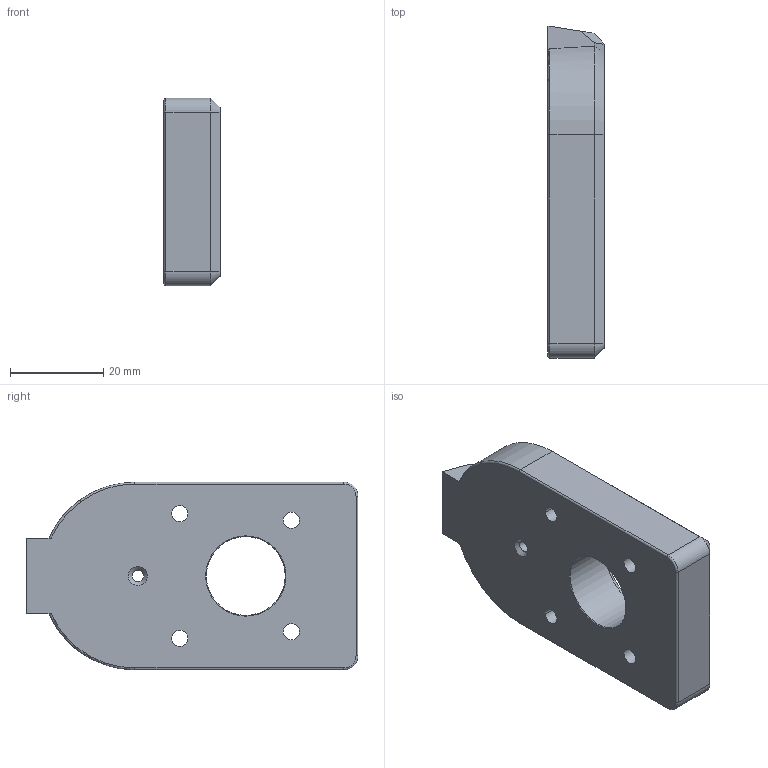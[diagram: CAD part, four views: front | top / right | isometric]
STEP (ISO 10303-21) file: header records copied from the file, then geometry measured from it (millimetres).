
FILE_DESCRIPTION (( 'STEP AP203' ), '1' );
FILE_NAME ('minimalist_barrel_retainer_cap.STEP', '2020-05-10T06:18:31', ( '' ), ( '' ), 'SwSTEP 2.0', 'SolidWorks 2016', '' );
FILE_SCHEMA (( 'CONFIG_CONTROL_DESIGN' ));
Length unit declared in the file: millimetre
Products named in the file (1): minimalist_barrel_retainer_cap
Bounding box: 12 x 71.08 x 40.2 mm (x, y, z)
Volume: 27410.1 mm3; surface area: 8116.6 mm2
Topology: 1 solids, 1 shells, 46 faces, 113 edges, 70 vertices
Faces by surface type: plane 19, cylinder 14, torus 6, cone 6, bspline 1
Full cylindrical faces by diameter (mm): 2.5 x2, 3.5 x2, 16.9 x1
Entity records: 1505 total; most frequent: CARTESIAN_POINT 352, DIRECTION 227, ORIENTED_EDGE 208, EDGE_CURVE 104, AXIS2_PLACEMENT_3D 86, VERTEX_POINT 69, EDGE_LOOP 67, LINE 55
